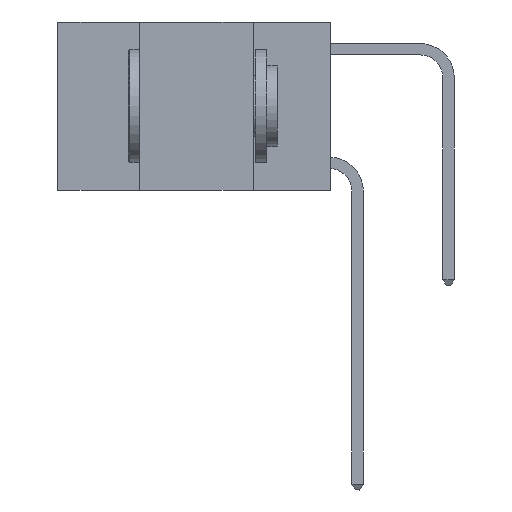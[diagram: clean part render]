
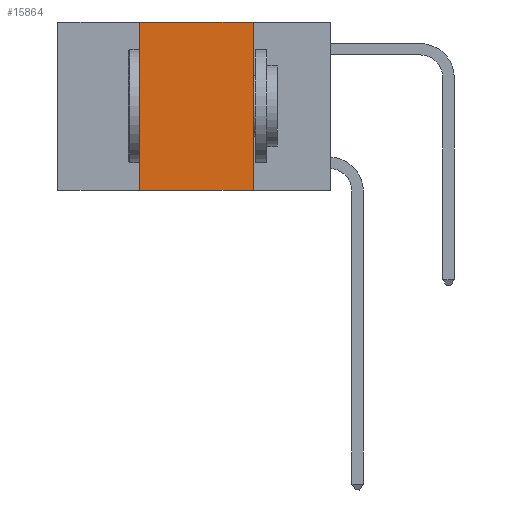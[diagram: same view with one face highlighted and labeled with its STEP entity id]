
A CAD part, left-side view. The second image highlights one B-rep face of the part: STEP entity #15864.
In plain terms, the highlighted planar face has unit normal (-1, 0, 0).
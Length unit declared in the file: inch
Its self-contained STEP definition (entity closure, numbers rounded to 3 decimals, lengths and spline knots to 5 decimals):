
#79 = CARTESIAN_POINT ( 'NONE',  ( 0., 0.17, 0. ) ) ;
#1802 = VECTOR ( 'NONE', #3162, 39.37008 ) ;
#2037 = EDGE_CURVE ( 'NONE', #20391, #14272, #18784, .T. ) ;
#2529 = VERTEX_POINT ( 'NONE', #6037 ) ;
#3162 = DIRECTION ( 'NONE',  ( 0., 0., 1. ) ) ;
#4237 = DIRECTION ( 'NONE',  ( 0., -1., 0. ) ) ;
#4621 = DIRECTION ( 'NONE',  ( 0., 0., -1. ) ) ;
#5483 = VECTOR ( 'NONE', #4621, 39.37008 ) ;
#6037 = CARTESIAN_POINT ( 'NONE',  ( 0., 0.42, -0.37 ) ) ;
#7128 = LINE ( 'NONE', #17031, #1802 ) ;
#7243 = VECTOR ( 'NONE', #4237, 39.37008 ) ;
#7896 = EDGE_CURVE ( 'NONE', #2529, #14272, #23796, .T. ) ;
#9855 = EDGE_LOOP ( 'NONE', ( #11731, #12044, #13997, #14921 ) ) ;
#11472 = VERTEX_POINT ( 'NONE', #17669 ) ;
#11583 = DIRECTION ( 'NONE',  ( 1., 0., 0. ) ) ;
#11731 = ORIENTED_EDGE ( 'NONE', *, *, #2037, .F. ) ;
#11857 = EDGE_CURVE ( 'NONE', #2529, #11472, #7128, .T. ) ;
#12044 = ORIENTED_EDGE ( 'NONE', *, *, #20787, .F. ) ;
#12495 = LINE ( 'NONE', #16009, #7243 ) ;
#12539 = VECTOR ( 'NONE', #25363, 39.37008 ) ;
#13997 = ORIENTED_EDGE ( 'NONE', *, *, #11857, .F. ) ;
#14272 = VERTEX_POINT ( 'NONE', #24009 ) ;
#14921 = ORIENTED_EDGE ( 'NONE', *, *, #7896, .T. ) ;
#15370 = CARTESIAN_POINT ( 'NONE',  ( 0., 0.6, -0.37 ) ) ;
#15864 = ADVANCED_FACE ( 'NONE', ( #21907 ), #19488, .F. ) ;
#16009 = CARTESIAN_POINT ( 'NONE',  ( 0., 0.6, 0. ) ) ;
#17031 = CARTESIAN_POINT ( 'NONE',  ( 0., 0.42, 0. ) ) ;
#17477 = CARTESIAN_POINT ( 'NONE',  ( 0., 0.6, 0. ) ) ;
#17669 = CARTESIAN_POINT ( 'NONE',  ( 0., 0.42, 0. ) ) ;
#18784 = LINE ( 'NONE', #79, #5483 ) ;
#19488 = PLANE ( 'NONE',  #25515 ) ;
#20391 = VERTEX_POINT ( 'NONE', #20944 ) ;
#20787 = EDGE_CURVE ( 'NONE', #11472, #20391, #12495, .T. ) ;
#20944 = CARTESIAN_POINT ( 'NONE',  ( 0., 0.17, 0. ) ) ;
#21907 = FACE_OUTER_BOUND ( 'NONE', #9855, .T. ) ;
#23796 = LINE ( 'NONE', #15370, #12539 ) ;
#24009 = CARTESIAN_POINT ( 'NONE',  ( 0., 0.17, -0.37 ) ) ;
#25363 = DIRECTION ( 'NONE',  ( 0., -1., 0. ) ) ;
#25515 = AXIS2_PLACEMENT_3D ( 'NONE', #17477, #11583, #25546 ) ;
#25546 = DIRECTION ( 'NONE',  ( 0., 0., -1. ) ) ;
